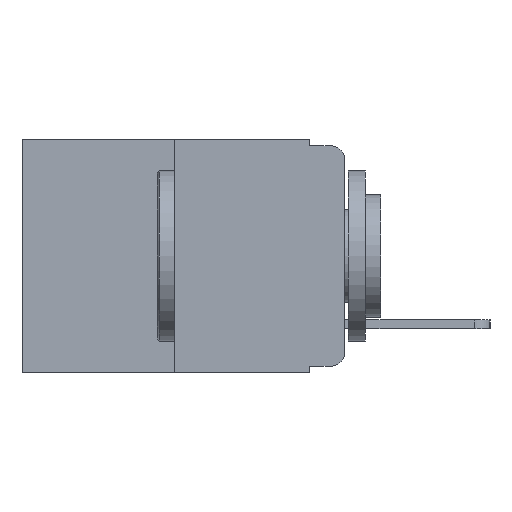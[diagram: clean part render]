
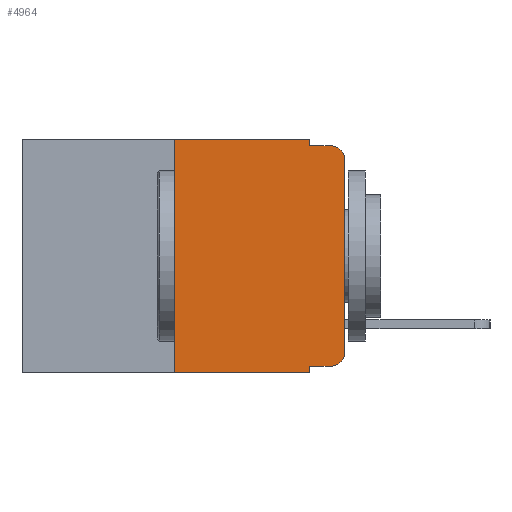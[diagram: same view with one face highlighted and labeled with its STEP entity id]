
A CAD part, left-side view. The second image highlights one B-rep face of the part: STEP entity #4964.
In plain terms, the highlighted planar face has unit normal (-1, 0, 0).
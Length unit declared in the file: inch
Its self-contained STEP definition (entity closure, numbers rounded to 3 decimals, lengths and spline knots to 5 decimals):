
#414 = CARTESIAN_POINT ( 'NONE',  ( 0., 0.051, -0.01 ) ) ;
#800 = EDGE_CURVE ( 'NONE', #14905, #6777, #10985, .T. ) ;
#1198 = VECTOR ( 'NONE', #10659, 39.37008 ) ;
#1345 = CARTESIAN_POINT ( 'NONE',  ( 0., 0.25, 0. ) ) ;
#2316 = ORIENTED_EDGE ( 'NONE', *, *, #14170, .F. ) ;
#2346 = CIRCLE ( 'NONE', #10873, 0.02 ) ;
#2889 = LINE ( 'NONE', #3663, #9889 ) ;
#3014 = EDGE_CURVE ( 'NONE', #6045, #13218, #13124, .T. ) ;
#3032 = EDGE_CURVE ( 'NONE', #13218, #8575, #15766, .T. ) ;
#3034 = EDGE_CURVE ( 'NONE', #3662, #8575, #8868, .T. ) ;
#3036 = EDGE_CURVE ( 'NONE', #10299, #3662, #5618, .T. ) ;
#3348 = LINE ( 'NONE', #10158, #16715 ) ;
#3366 = EDGE_CURVE ( 'NONE', #14905, #5239, #11126, .T. ) ;
#3381 = DIRECTION ( 'NONE',  ( 0., 0., -1. ) ) ;
#3403 = EDGE_CURVE ( 'NONE', #6545, #9134, #3348, .T. ) ;
#3406 = EDGE_CURVE ( 'NONE', #6545, #6777, #2889, .T. ) ;
#3435 = PLANE ( 'NONE',  #8121 ) ;
#3662 = VERTEX_POINT ( 'NONE', #414 ) ;
#3663 = CARTESIAN_POINT ( 'NONE',  ( 0., 0.051, 0. ) ) ;
#3724 = ORIENTED_EDGE ( 'NONE', *, *, #11523, .T. ) ;
#4052 = EDGE_LOOP ( 'NONE', ( #11254, #15448, #15891, #12826, #2316, #13227, #13619, #17028, #10665, #3724 ) ) ;
#4235 = CARTESIAN_POINT ( 'NONE',  ( 0., 0.051, 0. ) ) ;
#4287 = DIRECTION ( 'NONE',  ( 0., 0., -1. ) ) ;
#4391 = CARTESIAN_POINT ( 'NONE',  ( 0., 0.02, -0.333 ) ) ;
#4504 = DIRECTION ( 'NONE',  ( -1., 0., 0. ) ) ;
#4964 = ADVANCED_FACE ( 'NONE', ( #12285 ), #3435, .F. ) ;
#5085 = CARTESIAN_POINT ( 'NONE',  ( 0., 0.02, -0.03 ) ) ;
#5108 = CARTESIAN_POINT ( 'NONE',  ( 0., 0.051, -0.01 ) ) ;
#5239 = VERTEX_POINT ( 'NONE', #1345 ) ;
#5336 = CARTESIAN_POINT ( 'NONE',  ( 0., 0., 0. ) ) ;
#5458 = DIRECTION ( 'NONE',  ( 0., -1., 0. ) ) ;
#5618 = LINE ( 'NONE', #4235, #11925 ) ;
#6045 = VERTEX_POINT ( 'NONE', #14034 ) ;
#6089 = CARTESIAN_POINT ( 'NONE',  ( 0., 0.473, -0.343 ) ) ;
#6297 = CARTESIAN_POINT ( 'NONE',  ( 0., 0.051, 0. ) ) ;
#6545 = VERTEX_POINT ( 'NONE', #16700 ) ;
#6777 = VERTEX_POINT ( 'NONE', #16072 ) ;
#7007 = VECTOR ( 'NONE', #11006, 39.37008 ) ;
#7064 = CARTESIAN_POINT ( 'NONE',  ( 0., 0.25, 0. ) ) ;
#7426 = AXIS2_PLACEMENT_3D ( 'NONE', #5085, #4504, #4287 ) ;
#7454 = DIRECTION ( 'NONE',  ( 0., 0., 1. ) ) ;
#8104 = CARTESIAN_POINT ( 'NONE',  ( 0., 0.02, -0.313 ) ) ;
#8121 = AXIS2_PLACEMENT_3D ( 'NONE', #15517, #15620, #15616 ) ;
#8519 = DIRECTION ( 'NONE',  ( 0., -1., 0. ) ) ;
#8575 = VERTEX_POINT ( 'NONE', #13295 ) ;
#8868 = LINE ( 'NONE', #5108, #1198 ) ;
#9134 = VERTEX_POINT ( 'NONE', #4391 ) ;
#9423 = DIRECTION ( 'NONE',  ( 0., 0., -1. ) ) ;
#9835 = DIRECTION ( 'NONE',  ( 0., 0., 1. ) ) ;
#9889 = VECTOR ( 'NONE', #11088, 39.37008 ) ;
#9991 = VECTOR ( 'NONE', #5458, 39.37008 ) ;
#10118 = CARTESIAN_POINT ( 'NONE',  ( 0., 0., -0.03 ) ) ;
#10158 = CARTESIAN_POINT ( 'NONE',  ( 0., 0.051, -0.333 ) ) ;
#10299 = VERTEX_POINT ( 'NONE', #6297 ) ;
#10659 = DIRECTION ( 'NONE',  ( 0., -1., 0. ) ) ;
#10665 = ORIENTED_EDGE ( 'NONE', *, *, #3403, .T. ) ;
#10873 = AXIS2_PLACEMENT_3D ( 'NONE', #8104, #17112, #9423 ) ;
#10985 = LINE ( 'NONE', #6089, #7007 ) ;
#11006 = DIRECTION ( 'NONE',  ( 0., -1., 0. ) ) ;
#11088 = DIRECTION ( 'NONE',  ( 0., 0., -1. ) ) ;
#11126 = LINE ( 'NONE', #7064, #17439 ) ;
#11254 = ORIENTED_EDGE ( 'NONE', *, *, #3014, .T. ) ;
#11523 = EDGE_CURVE ( 'NONE', #9134, #6045, #2346, .T. ) ;
#11925 = VECTOR ( 'NONE', #3381, 39.37008 ) ;
#12285 = FACE_OUTER_BOUND ( 'NONE', #4052, .T. ) ;
#12826 = ORIENTED_EDGE ( 'NONE', *, *, #3036, .F. ) ;
#13124 = LINE ( 'NONE', #5336, #16925 ) ;
#13218 = VERTEX_POINT ( 'NONE', #10118 ) ;
#13227 = ORIENTED_EDGE ( 'NONE', *, *, #3366, .F. ) ;
#13295 = CARTESIAN_POINT ( 'NONE',  ( 0., 0.02, -0.01 ) ) ;
#13374 = LINE ( 'NONE', #16015, #9991 ) ;
#13619 = ORIENTED_EDGE ( 'NONE', *, *, #800, .T. ) ;
#14034 = CARTESIAN_POINT ( 'NONE',  ( 0., 0., -0.313 ) ) ;
#14170 = EDGE_CURVE ( 'NONE', #5239, #10299, #13374, .T. ) ;
#14751 = CARTESIAN_POINT ( 'NONE',  ( 0., 0.25, -0.343 ) ) ;
#14905 = VERTEX_POINT ( 'NONE', #14751 ) ;
#15448 = ORIENTED_EDGE ( 'NONE', *, *, #3032, .T. ) ;
#15517 = CARTESIAN_POINT ( 'NONE',  ( 0., 0.473, 0. ) ) ;
#15616 = DIRECTION ( 'NONE',  ( 0., 0., -1. ) ) ;
#15620 = DIRECTION ( 'NONE',  ( 1., 0., 0. ) ) ;
#15766 = CIRCLE ( 'NONE', #7426, 0.02 ) ;
#15891 = ORIENTED_EDGE ( 'NONE', *, *, #3034, .F. ) ;
#16015 = CARTESIAN_POINT ( 'NONE',  ( 0., 0.473, 0. ) ) ;
#16072 = CARTESIAN_POINT ( 'NONE',  ( 0., 0.051, -0.343 ) ) ;
#16700 = CARTESIAN_POINT ( 'NONE',  ( 0., 0.051, -0.333 ) ) ;
#16715 = VECTOR ( 'NONE', #8519, 39.37008 ) ;
#16925 = VECTOR ( 'NONE', #7454, 39.37008 ) ;
#17028 = ORIENTED_EDGE ( 'NONE', *, *, #3406, .F. ) ;
#17112 = DIRECTION ( 'NONE',  ( -1., 0., 0. ) ) ;
#17439 = VECTOR ( 'NONE', #9835, 39.37008 ) ;
